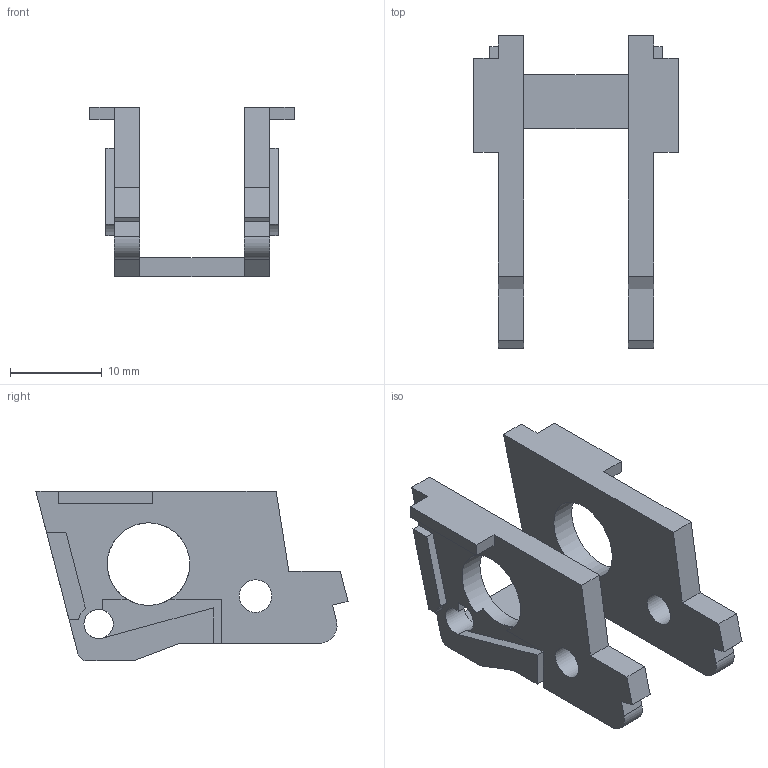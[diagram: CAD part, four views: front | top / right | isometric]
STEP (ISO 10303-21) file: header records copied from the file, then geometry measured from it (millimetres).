
FILE_DESCRIPTION(/* description */ (''),/* implementation_level */ '2;1');
FILE_NAME(/* name */ 'Locking Block.step',/* time_stamp */ '2021-03-06T17:01:29-05:00',/* author */ (''),/* organization */ (''),/* preprocessor_version */ 'ST-DEVELOPER v18.1',/* originating_system */ 'Autodesk Translation Framework v9.10.0.1330',/* authorisation */ '');
FILE_SCHEMA (('AUTOMOTIVE_DESIGN { 1 0 10303 214 3 1 1 }'));
Length unit declared in the file: millimetre
Products named in the file (1): Locking Block
Bounding box: 22.3 x 34.03 x 18.5 mm (x, y, z)
Volume: 2377.1 mm3; surface area: 2718.7 mm2
Topology: 1 solids, 1 shells, 58 faces, 174 edges, 116 vertices
Faces by surface type: plane 47, cylinder 11
Full cylindrical faces by diameter (mm): 3.2 x2, 3.55 x2, 9 x2
Entity records: 2001 total; most frequent: CARTESIAN_POINT 349, ORIENTED_EDGE 348, DIRECTION 318, EDGE_CURVE 174, LINE 148, VECTOR 148, VERTEX_POINT 116, AXIS2_PLACEMENT_3D 85
